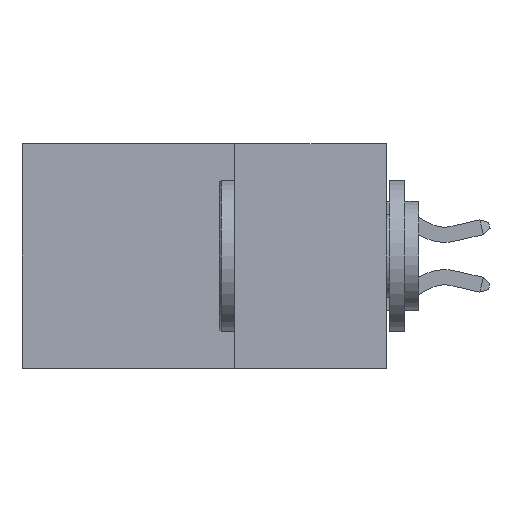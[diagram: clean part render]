
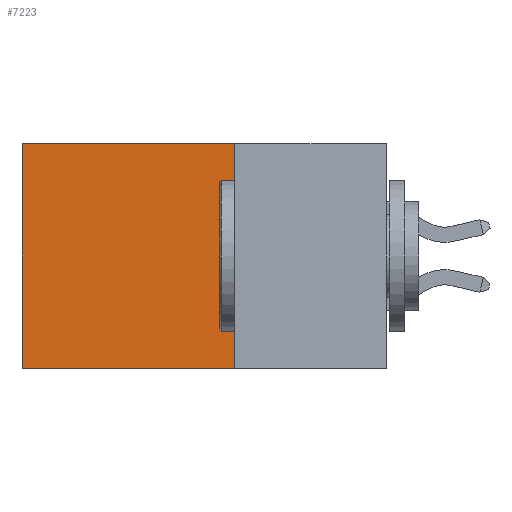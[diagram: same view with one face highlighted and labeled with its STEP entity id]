
A CAD part, left-side view. The second image highlights one B-rep face of the part: STEP entity #7223.
In plain terms, the highlighted planar face has unit normal (-1, 0, 0).
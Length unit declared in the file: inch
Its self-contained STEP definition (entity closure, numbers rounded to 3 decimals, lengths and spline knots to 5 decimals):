
#168 = DIRECTION ( 'NONE',  ( 0., 1., 0. ) ) ;
#1235 = DIRECTION ( 'NONE',  ( 1., 0., 0. ) ) ;
#2962 = LINE ( 'NONE', #4122, #5860 ) ;
#3115 = ORIENTED_EDGE ( 'NONE', *, *, #5636, .T. ) ;
#3789 = CARTESIAN_POINT ( 'NONE',  ( 0.298, 0.25, -0.37 ) ) ;
#3986 = VERTEX_POINT ( 'NONE', #7250 ) ;
#4014 = DIRECTION ( 'NONE',  ( 0., 0., -1. ) ) ;
#4122 = CARTESIAN_POINT ( 'NONE',  ( 0.298, 0.25, 0. ) ) ;
#4789 = CARTESIAN_POINT ( 'NONE',  ( 0.298, 0.25, 0. ) ) ;
#4912 = CARTESIAN_POINT ( 'NONE',  ( 0.298, 0.25, 0. ) ) ;
#5286 = LINE ( 'NONE', #7898, #11581 ) ;
#5357 = EDGE_CURVE ( 'NONE', #9864, #15255, #2962, .T. ) ;
#5636 = EDGE_CURVE ( 'NONE', #8277, #3986, #5286, .T. ) ;
#5860 = VECTOR ( 'NONE', #4014, 39.37008 ) ;
#6921 = AXIS2_PLACEMENT_3D ( 'NONE', #4912, #1235, #9711 ) ;
#7128 = CARTESIAN_POINT ( 'NONE',  ( 0.298, 0.25, 0. ) ) ;
#7223 = ADVANCED_FACE ( 'NONE', ( #14428 ), #8537, .F. ) ;
#7239 = VECTOR ( 'NONE', #168, 39.37008 ) ;
#7250 = CARTESIAN_POINT ( 'NONE',  ( 0.298, 0.6, -0.37 ) ) ;
#7898 = CARTESIAN_POINT ( 'NONE',  ( 0.298, 0.6, 0. ) ) ;
#8277 = VERTEX_POINT ( 'NONE', #9932 ) ;
#8537 = PLANE ( 'NONE',  #6921 ) ;
#8629 = ORIENTED_EDGE ( 'NONE', *, *, #12839, .F. ) ;
#9102 = EDGE_LOOP ( 'NONE', ( #3115, #8629, #10629, #11426 ) ) ;
#9711 = DIRECTION ( 'NONE',  ( 0., 0., -1. ) ) ;
#9771 = DIRECTION ( 'NONE',  ( 0., 0., -1. ) ) ;
#9864 = VERTEX_POINT ( 'NONE', #7128 ) ;
#9932 = CARTESIAN_POINT ( 'NONE',  ( 0.298, 0.6, 0. ) ) ;
#10224 = LINE ( 'NONE', #4789, #13311 ) ;
#10360 = LINE ( 'NONE', #3789, #7239 ) ;
#10629 = ORIENTED_EDGE ( 'NONE', *, *, #5357, .F. ) ;
#11426 = ORIENTED_EDGE ( 'NONE', *, *, #14790, .T. ) ;
#11581 = VECTOR ( 'NONE', #9771, 39.37008 ) ;
#12839 = EDGE_CURVE ( 'NONE', #15255, #3986, #10360, .T. ) ;
#13311 = VECTOR ( 'NONE', #14160, 39.37008 ) ;
#14046 = CARTESIAN_POINT ( 'NONE',  ( 0.298, 0.25, -0.37 ) ) ;
#14160 = DIRECTION ( 'NONE',  ( 0., 1., 0. ) ) ;
#14428 = FACE_OUTER_BOUND ( 'NONE', #9102, .T. ) ;
#14790 = EDGE_CURVE ( 'NONE', #9864, #8277, #10224, .T. ) ;
#15255 = VERTEX_POINT ( 'NONE', #14046 ) ;
